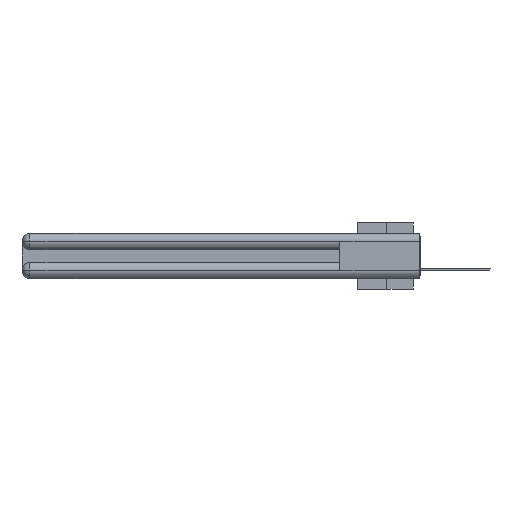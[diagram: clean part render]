
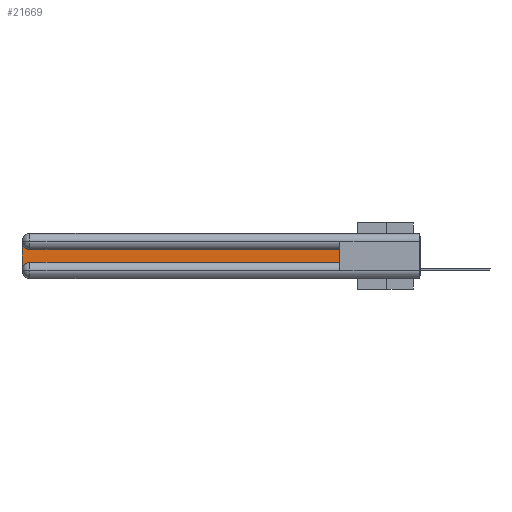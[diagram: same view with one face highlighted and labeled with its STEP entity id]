
A CAD part, left-side view. The second image highlights one B-rep face of the part: STEP entity #21669.
In plain terms, the highlighted planar face has unit normal (-1, 0, 0).
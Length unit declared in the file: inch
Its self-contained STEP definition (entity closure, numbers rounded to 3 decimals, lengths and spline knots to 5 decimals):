
#59 = AXIS2_PLACEMENT_3D ( 'NONE', #5223, #2535, #22967 ) ;
#1481 = LINE ( 'NONE', #22469, #16569 ) ;
#1926 = DIRECTION ( 'NONE',  ( 0., 0., -1. ) ) ;
#2014 = DIRECTION ( 'NONE',  ( 0., 0., -1. ) ) ;
#2535 = DIRECTION ( 'NONE',  ( 1., 0., 0. ) ) ;
#2945 = VECTOR ( 'NONE', #17038, 39.37008 ) ;
#3188 = CARTESIAN_POINT ( 'NONE',  ( 0.075, 2.94, -0.1225 ) ) ;
#3262 = CARTESIAN_POINT ( 'NONE',  ( 0.075, 3., -0.0625 ) ) ;
#4659 = VERTEX_POINT ( 'NONE', #31534 ) ;
#4774 = CIRCLE ( 'NONE', #59, 0.06 ) ;
#4805 = CIRCLE ( 'NONE', #33271, 0.06 ) ;
#5008 = AXIS2_PLACEMENT_3D ( 'NONE', #19400, #19531, #2014 ) ;
#5223 = CARTESIAN_POINT ( 'NONE',  ( 0.075, 2.94, -0.2775 ) ) ;
#5881 = CARTESIAN_POINT ( 'NONE',  ( 0.075, 0.6, -0.1225 ) ) ;
#7077 = CARTESIAN_POINT ( 'NONE',  ( 0.075, 0.6, -0.1225 ) ) ;
#7158 = DIRECTION ( 'NONE',  ( 1., 0., 0. ) ) ;
#7636 = PLANE ( 'NONE',  #5008 ) ;
#9023 = CARTESIAN_POINT ( 'NONE',  ( 0.075, 0.6, -0.2175 ) ) ;
#10182 = EDGE_CURVE ( 'NONE', #35161, #4659, #1481, .T. ) ;
#10473 = DIRECTION ( 'NONE',  ( 0., 0., -1. ) ) ;
#10841 = ORIENTED_EDGE ( 'NONE', *, *, #11430, .T. ) ;
#11430 = EDGE_CURVE ( 'NONE', #22275, #34468, #34887, .T. ) ;
#14153 = CARTESIAN_POINT ( 'NONE',  ( 0.075, 0.6, -0.2175 ) ) ;
#16569 = VECTOR ( 'NONE', #1926, 39.37008 ) ;
#16841 = EDGE_CURVE ( 'NONE', #34468, #35161, #4805, .T. ) ;
#16963 = VECTOR ( 'NONE', #32061, 39.37008 ) ;
#17038 = DIRECTION ( 'NONE',  ( 0., -1., 0. ) ) ;
#17129 = VERTEX_POINT ( 'NONE', #14153 ) ;
#17169 = ORIENTED_EDGE ( 'NONE', *, *, #21162, .T. ) ;
#18350 = CARTESIAN_POINT ( 'NONE',  ( 0.075, 2.94, -0.2175 ) ) ;
#18713 = EDGE_LOOP ( 'NONE', ( #10841, #35067, #22901, #28019, #24332, #17169 ) ) ;
#19400 = CARTESIAN_POINT ( 'NONE',  ( 0.075, 3., -0.1225 ) ) ;
#19531 = DIRECTION ( 'NONE',  ( 1., 0., 0. ) ) ;
#21162 = EDGE_CURVE ( 'NONE', #17129, #22275, #35764, .T. ) ;
#21384 = VERTEX_POINT ( 'NONE', #18350 ) ;
#21669 = ADVANCED_FACE ( 'NONE', ( #24242 ), #7636, .F. ) ;
#22275 = VERTEX_POINT ( 'NONE', #5881 ) ;
#22469 = CARTESIAN_POINT ( 'NONE',  ( 0.075, 3., -0.2175 ) ) ;
#22901 = ORIENTED_EDGE ( 'NONE', *, *, #10182, .T. ) ;
#22967 = DIRECTION ( 'NONE',  ( 0., 0., -1. ) ) ;
#23057 = CARTESIAN_POINT ( 'NONE',  ( 0.075, 0.6, -0.2175 ) ) ;
#24242 = FACE_OUTER_BOUND ( 'NONE', #18713, .T. ) ;
#24332 = ORIENTED_EDGE ( 'NONE', *, *, #30867, .T. ) ;
#24386 = LINE ( 'NONE', #23057, #2945 ) ;
#24640 = CARTESIAN_POINT ( 'NONE',  ( 0.075, 2.94, -0.0625 ) ) ;
#27091 = VECTOR ( 'NONE', #35718, 39.37008 ) ;
#28019 = ORIENTED_EDGE ( 'NONE', *, *, #37293, .T. ) ;
#30867 = EDGE_CURVE ( 'NONE', #21384, #17129, #24386, .T. ) ;
#31534 = CARTESIAN_POINT ( 'NONE',  ( 0.075, 3., -0.2775 ) ) ;
#32061 = DIRECTION ( 'NONE',  ( 0., 0., 1. ) ) ;
#33271 = AXIS2_PLACEMENT_3D ( 'NONE', #24640, #7158, #10473 ) ;
#34468 = VERTEX_POINT ( 'NONE', #3188 ) ;
#34887 = LINE ( 'NONE', #7077, #27091 ) ;
#35067 = ORIENTED_EDGE ( 'NONE', *, *, #16841, .T. ) ;
#35161 = VERTEX_POINT ( 'NONE', #3262 ) ;
#35718 = DIRECTION ( 'NONE',  ( 0., 1., 0. ) ) ;
#35764 = LINE ( 'NONE', #9023, #16963 ) ;
#37293 = EDGE_CURVE ( 'NONE', #4659, #21384, #4774, .T. ) ;
